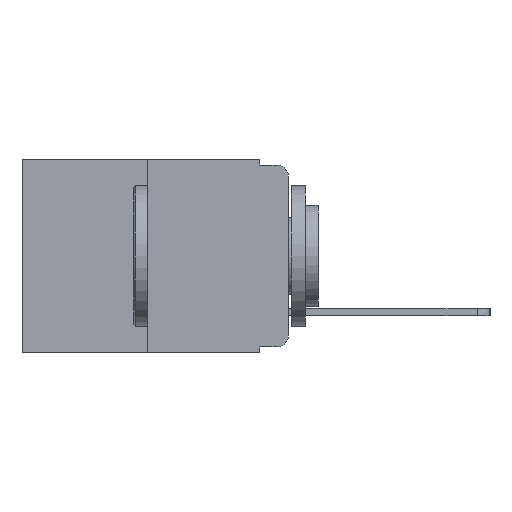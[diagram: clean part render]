
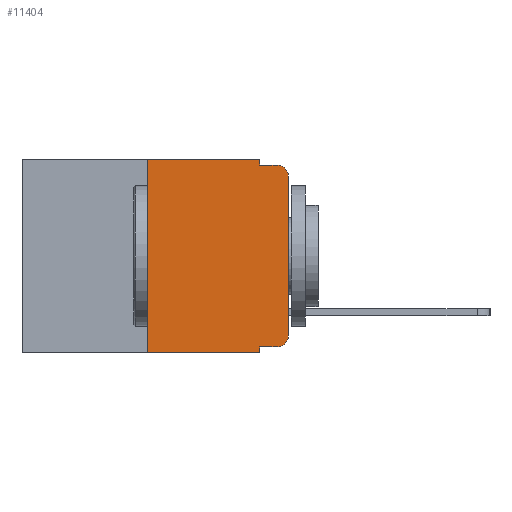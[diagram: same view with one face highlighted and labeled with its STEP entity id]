
A CAD part, left-side view. The second image highlights one B-rep face of the part: STEP entity #11404.
In plain terms, the highlighted planar face has unit normal (-1, 0, 0).
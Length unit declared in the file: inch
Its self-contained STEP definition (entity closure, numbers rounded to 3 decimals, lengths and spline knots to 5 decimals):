
#34 = PLANE ( 'NONE',  #11841 ) ;
#620 = CIRCLE ( 'NONE', #18562, 0.02 ) ;
#924 = FACE_OUTER_BOUND ( 'NONE', #15605, .T. ) ;
#1327 = CARTESIAN_POINT ( 'NONE',  ( 0., 0.051, -0.01 ) ) ;
#1354 = DIRECTION ( 'NONE',  ( 0., 0., 1. ) ) ;
#1486 = CARTESIAN_POINT ( 'NONE',  ( 0., 0.25, 0. ) ) ;
#1697 = CARTESIAN_POINT ( 'NONE',  ( 0., 0.02, -0.333 ) ) ;
#2094 = CARTESIAN_POINT ( 'NONE',  ( 0., 0.473, -0.343 ) ) ;
#2147 = VECTOR ( 'NONE', #14414, 39.37008 ) ;
#2317 = LINE ( 'NONE', #12492, #17538 ) ;
#2635 = LINE ( 'NONE', #1486, #10862 ) ;
#2707 = AXIS2_PLACEMENT_3D ( 'NONE', #13799, #5071, #15200 ) ;
#3045 = EDGE_CURVE ( 'NONE', #13913, #4442, #2635, .T. ) ;
#3469 = CARTESIAN_POINT ( 'NONE',  ( 0., 0.02, -0.313 ) ) ;
#3774 = LINE ( 'NONE', #2094, #18693 ) ;
#3961 = CARTESIAN_POINT ( 'NONE',  ( 0., 0., -0.313 ) ) ;
#4110 = CARTESIAN_POINT ( 'NONE',  ( 0., 0.051, -0.333 ) ) ;
#4427 = VERTEX_POINT ( 'NONE', #1327 ) ;
#4442 = VERTEX_POINT ( 'NONE', #15986 ) ;
#4632 = EDGE_CURVE ( 'NONE', #7122, #4427, #2317, .T. ) ;
#4716 = VERTEX_POINT ( 'NONE', #15892 ) ;
#4918 = EDGE_CURVE ( 'NONE', #6838, #16972, #10567, .T. ) ;
#5071 = DIRECTION ( 'NONE',  ( -1., 0., 0. ) ) ;
#5122 = DIRECTION ( 'NONE',  ( 0., 0., -1. ) ) ;
#5132 = EDGE_CURVE ( 'NONE', #13435, #4716, #11444, .T. ) ;
#5139 = DIRECTION ( 'NONE',  ( 0., 0., -1. ) ) ;
#5264 = DIRECTION ( 'NONE',  ( 0., 0., 1. ) ) ;
#5510 = ORIENTED_EDGE ( 'NONE', *, *, #13965, .T. ) ;
#6329 = EDGE_CURVE ( 'NONE', #4427, #16972, #7162, .T. ) ;
#6620 = LINE ( 'NONE', #18046, #13864 ) ;
#6780 = VERTEX_POINT ( 'NONE', #1697 ) ;
#6838 = VERTEX_POINT ( 'NONE', #11126 ) ;
#7122 = VERTEX_POINT ( 'NONE', #14429 ) ;
#7162 = LINE ( 'NONE', #10134, #17615 ) ;
#7680 = VECTOR ( 'NONE', #9743, 39.37008 ) ;
#7965 = EDGE_CURVE ( 'NONE', #18327, #6838, #6620, .T. ) ;
#8141 = ORIENTED_EDGE ( 'NONE', *, *, #13106, .F. ) ;
#9743 = DIRECTION ( 'NONE',  ( 0., -1., 0. ) ) ;
#9991 = DIRECTION ( 'NONE',  ( 0., -1., 0. ) ) ;
#10032 = ORIENTED_EDGE ( 'NONE', *, *, #3045, .F. ) ;
#10134 = CARTESIAN_POINT ( 'NONE',  ( 0., 0.051, -0.01 ) ) ;
#10567 = CIRCLE ( 'NONE', #2707, 0.02 ) ;
#10862 = VECTOR ( 'NONE', #1354, 39.37008 ) ;
#10903 = LINE ( 'NONE', #12980, #2147 ) ;
#11009 = VECTOR ( 'NONE', #18671, 39.37008 ) ;
#11126 = CARTESIAN_POINT ( 'NONE',  ( 0., 0., -0.03 ) ) ;
#11404 = ADVANCED_FACE ( 'NONE', ( #924 ), #34, .F. ) ;
#11444 = LINE ( 'NONE', #14609, #11009 ) ;
#11841 = AXIS2_PLACEMENT_3D ( 'NONE', #16584, #13841, #5122 ) ;
#12308 = DIRECTION ( 'NONE',  ( 0., 0., -1. ) ) ;
#12492 = CARTESIAN_POINT ( 'NONE',  ( 0., 0.051, 0. ) ) ;
#12714 = CARTESIAN_POINT ( 'NONE',  ( 0., 0.02, -0.01 ) ) ;
#12980 = CARTESIAN_POINT ( 'NONE',  ( 0., 0.051, -0.333 ) ) ;
#13042 = EDGE_CURVE ( 'NONE', #6780, #18327, #620, .T. ) ;
#13062 = ORIENTED_EDGE ( 'NONE', *, *, #5132, .F. ) ;
#13106 = EDGE_CURVE ( 'NONE', #4442, #7122, #15282, .T. ) ;
#13435 = VERTEX_POINT ( 'NONE', #4110 ) ;
#13799 = CARTESIAN_POINT ( 'NONE',  ( 0., 0.02, -0.03 ) ) ;
#13841 = DIRECTION ( 'NONE',  ( 1., 0., 0. ) ) ;
#13855 = DIRECTION ( 'NONE',  ( -1., 0., 0. ) ) ;
#13864 = VECTOR ( 'NONE', #5264, 39.37008 ) ;
#13913 = VERTEX_POINT ( 'NONE', #16826 ) ;
#13965 = EDGE_CURVE ( 'NONE', #13913, #4716, #3774, .T. ) ;
#14038 = EDGE_CURVE ( 'NONE', #13435, #6780, #10903, .T. ) ;
#14414 = DIRECTION ( 'NONE',  ( 0., -1., 0. ) ) ;
#14429 = CARTESIAN_POINT ( 'NONE',  ( 0., 0.051, 0. ) ) ;
#14609 = CARTESIAN_POINT ( 'NONE',  ( 0., 0.051, 0. ) ) ;
#15200 = DIRECTION ( 'NONE',  ( 0., 0., -1. ) ) ;
#15282 = LINE ( 'NONE', #18010, #7680 ) ;
#15605 = EDGE_LOOP ( 'NONE', ( #18482, #18512, #16180, #17642, #8141, #10032, #5510, #13062, #16108, #18674 ) ) ;
#15892 = CARTESIAN_POINT ( 'NONE',  ( 0., 0.051, -0.343 ) ) ;
#15986 = CARTESIAN_POINT ( 'NONE',  ( 0., 0.25, 0. ) ) ;
#16108 = ORIENTED_EDGE ( 'NONE', *, *, #14038, .T. ) ;
#16180 = ORIENTED_EDGE ( 'NONE', *, *, #6329, .F. ) ;
#16584 = CARTESIAN_POINT ( 'NONE',  ( 0., 0.473, 0. ) ) ;
#16826 = CARTESIAN_POINT ( 'NONE',  ( 0., 0.25, -0.343 ) ) ;
#16972 = VERTEX_POINT ( 'NONE', #12714 ) ;
#17088 = DIRECTION ( 'NONE',  ( 0., -1., 0. ) ) ;
#17538 = VECTOR ( 'NONE', #12308, 39.37008 ) ;
#17615 = VECTOR ( 'NONE', #17088, 39.37008 ) ;
#17642 = ORIENTED_EDGE ( 'NONE', *, *, #4632, .F. ) ;
#18010 = CARTESIAN_POINT ( 'NONE',  ( 0., 0.473, 0. ) ) ;
#18046 = CARTESIAN_POINT ( 'NONE',  ( 0., 0., 0. ) ) ;
#18327 = VERTEX_POINT ( 'NONE', #3961 ) ;
#18482 = ORIENTED_EDGE ( 'NONE', *, *, #7965, .T. ) ;
#18512 = ORIENTED_EDGE ( 'NONE', *, *, #4918, .T. ) ;
#18562 = AXIS2_PLACEMENT_3D ( 'NONE', #3469, #13855, #5139 ) ;
#18671 = DIRECTION ( 'NONE',  ( 0., 0., -1. ) ) ;
#18674 = ORIENTED_EDGE ( 'NONE', *, *, #13042, .T. ) ;
#18693 = VECTOR ( 'NONE', #9991, 39.37008 ) ;
